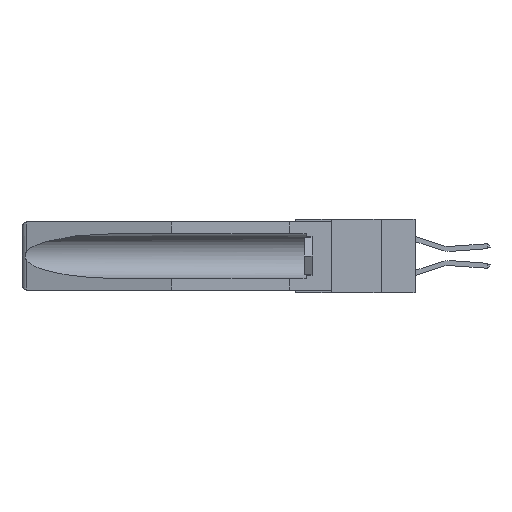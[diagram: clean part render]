
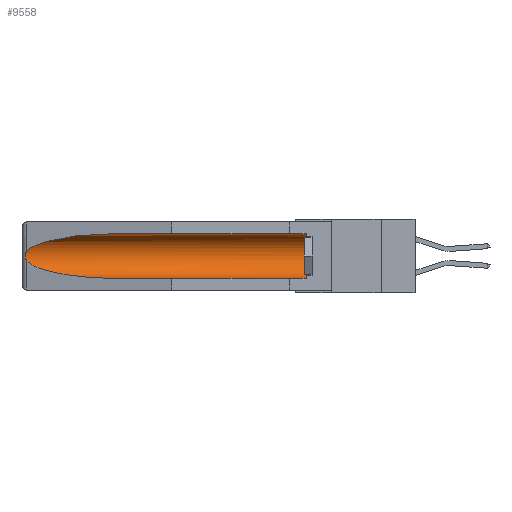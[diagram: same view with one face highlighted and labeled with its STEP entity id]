
A CAD part, left-side view. The second image highlights one B-rep face of the part: STEP entity #9558.
In plain terms, the highlighted cylindrical face has radius 2.857 mm (diameter 5.715 mm), a partial arc.
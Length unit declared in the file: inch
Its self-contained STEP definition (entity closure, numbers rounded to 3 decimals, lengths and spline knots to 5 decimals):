
#651 = ORIENTED_EDGE ( 'NONE', *, *, #10218, .F. ) ;
#733 = CIRCLE ( 'NONE', #18946, 0.1125 ) ;
#975 = CARTESIAN_POINT ( 'NONE',  ( 0.155, 1.07973, -0.059 ) ) ;
#1081 = CARTESIAN_POINT ( 'NONE',  ( 0.155, -0.30754, -0.1715 ) ) ;
#1108 = CARTESIAN_POINT ( 'NONE',  ( 0.155, 0.126, -0.284 ) ) ;
#1330 = VECTOR ( 'NONE', #5319, 39.37008 ) ;
#1684 = VERTEX_POINT ( 'NONE', #7099 ) ;
#2034 = CARTESIAN_POINT ( 'NONE',  ( 0.26537, 1.52718, -0.19328 ) ) ;
#2646 = DIRECTION ( 'NONE',  ( 0., 0., 1. ) ) ;
#2997 = CARTESIAN_POINT ( 'NONE',  ( 0.155, 0.126, -0.1715 ) ) ;
#3267 = EDGE_LOOP ( 'NONE', ( #19326, #18221, #10619, #651, #4637, #14459 ) ) ;
#3808 = CARTESIAN_POINT ( 'NONE',  ( 0.26537, 1.52718, -0.14972 ) ) ;
#3849 = DIRECTION ( 'NONE',  ( 0., 1., 0. ) ) ;
#4159 = EDGE_CURVE ( 'NONE', #10867, #6230, #10874, .T. ) ;
#4367 = CARTESIAN_POINT ( 'NONE',  ( 0.2675, 1.53308, -0.16763 ) ) ;
#4631 = DIRECTION ( 'NONE',  ( 0., 0., 1. ) ) ;
#4637 = ORIENTED_EDGE ( 'NONE', *, *, #15136, .T. ) ;
#5319 = DIRECTION ( 'NONE',  ( 0., 1., 0. ) ) ;
#5384 = CARTESIAN_POINT ( 'NONE',  ( 0.155, 1.07973, -0.059 ) ) ;
#5435 = EDGE_CURVE ( 'NONE', #6230, #8891, #6305, .T. ) ;
#5699 = CARTESIAN_POINT ( 'NONE',  ( 0.21114, 1.30732, -0.059 ) ) ;
#6230 = VERTEX_POINT ( 'NONE', #3808 ) ;
#6305 = B_SPLINE_CURVE_WITH_KNOTS ( 'NONE', 3,
 ( #15236, #7672, #13811, #8909, #4367, #15377, #16901, #19942, #10525, #20005 ),
 .UNSPECIFIED., .F., .F.,
 ( 4, 2, 2, 2, 4 ),
 ( 0., 0.00029, 0.00058, 0.00087, 0.00117 ),
 .UNSPECIFIED. ) ;
#7099 = CARTESIAN_POINT ( 'NONE',  ( 0.155, 0.126, -0.059 ) ) ;
#7160 = CARTESIAN_POINT ( 'NONE',  ( 0.155, -0.30754, -0.284 ) ) ;
#7672 = CARTESIAN_POINT ( 'NONE',  ( 0.26597, 1.52961, -0.15275 ) ) ;
#7878 = VERTEX_POINT ( 'NONE', #1108 ) ;
#8292 = CARTESIAN_POINT ( 'NONE',  ( 0.155, -0.30754, -0.059 ) ) ;
#8573 = CYLINDRICAL_SURFACE ( 'NONE', #11892, 0.1125 ) ;
#8720 =( BOUNDED_CURVE ( )  B_SPLINE_CURVE ( 3, ( #2034, #14272, #9805, #17841 ),
 .UNSPECIFIED., .F., .F. ) 
 B_SPLINE_CURVE_WITH_KNOTS ( ( 4, 4 ),
 ( 0.1948, 1.5708 ),
 .UNSPECIFIED. ) 
 CURVE ( )  GEOMETRIC_REPRESENTATION_ITEM ( )  RATIONAL_B_SPLINE_CURVE ( ( 1., 0.848, 0.848, 1. ) ) 
 REPRESENTATION_ITEM ( '' )  );
#8891 = VERTEX_POINT ( 'NONE', #19008 ) ;
#8909 = CARTESIAN_POINT ( 'NONE',  ( 0.2673, 1.5327, -0.16383 ) ) ;
#9558 = ADVANCED_FACE ( 'NONE', ( #14722 ), #8573, .F. ) ;
#9805 = CARTESIAN_POINT ( 'NONE',  ( 0.21114, 1.30732, -0.284 ) ) ;
#10205 = LINE ( 'NONE', #8292, #1330 ) ;
#10218 = EDGE_CURVE ( 'NONE', #7878, #10539, #19918, .T. ) ;
#10525 = CARTESIAN_POINT ( 'NONE',  ( 0.26597, 1.5296, -0.19026 ) ) ;
#10539 = VERTEX_POINT ( 'NONE', #16199 ) ;
#10619 = ORIENTED_EDGE ( 'NONE', *, *, #16459, .T. ) ;
#10867 = VERTEX_POINT ( 'NONE', #5384 ) ;
#10874 =( BOUNDED_CURVE ( )  B_SPLINE_CURVE ( 3, ( #975, #5699, #19913, #13640 ),
 .UNSPECIFIED., .F., .F. ) 
 B_SPLINE_CURVE_WITH_KNOTS ( ( 4, 4 ),
 ( 4.71239, 6.08839 ),
 .UNSPECIFIED. ) 
 CURVE ( )  GEOMETRIC_REPRESENTATION_ITEM ( )  RATIONAL_B_SPLINE_CURVE ( ( 1., 0.848, 0.848, 1. ) ) 
 REPRESENTATION_ITEM ( '' )  );
#11892 = AXIS2_PLACEMENT_3D ( 'NONE', #1081, #18478, #2646 ) ;
#11923 = VECTOR ( 'NONE', #3849, 39.37008 ) ;
#12382 = EDGE_CURVE ( 'NONE', #1684, #10867, #10205, .T. ) ;
#12521 = DIRECTION ( 'NONE',  ( 0., -1., 0. ) ) ;
#13640 = CARTESIAN_POINT ( 'NONE',  ( 0.26537, 1.52718, -0.14972 ) ) ;
#13811 = CARTESIAN_POINT ( 'NONE',  ( 0.26654, 1.53092, -0.15636 ) ) ;
#14272 = CARTESIAN_POINT ( 'NONE',  ( 0.25451, 1.48313, -0.24835 ) ) ;
#14459 = ORIENTED_EDGE ( 'NONE', *, *, #12382, .T. ) ;
#14722 = FACE_OUTER_BOUND ( 'NONE', #3267, .T. ) ;
#15136 = EDGE_CURVE ( 'NONE', #7878, #1684, #733, .T. ) ;
#15236 = CARTESIAN_POINT ( 'NONE',  ( 0.26537, 1.52718, -0.14972 ) ) ;
#15377 = CARTESIAN_POINT ( 'NONE',  ( 0.2675, 1.53308, -0.17534 ) ) ;
#16199 = CARTESIAN_POINT ( 'NONE',  ( 0.155, 1.07973, -0.284 ) ) ;
#16459 = EDGE_CURVE ( 'NONE', #8891, #10539, #8720, .T. ) ;
#16901 = CARTESIAN_POINT ( 'NONE',  ( 0.2673, 1.53269, -0.17917 ) ) ;
#17841 = CARTESIAN_POINT ( 'NONE',  ( 0.155, 1.07973, -0.284 ) ) ;
#18221 = ORIENTED_EDGE ( 'NONE', *, *, #5435, .T. ) ;
#18478 = DIRECTION ( 'NONE',  ( 0., 1., 0. ) ) ;
#18946 = AXIS2_PLACEMENT_3D ( 'NONE', #2997, #12521, #4631 ) ;
#19008 = CARTESIAN_POINT ( 'NONE',  ( 0.26537, 1.52718, -0.19328 ) ) ;
#19326 = ORIENTED_EDGE ( 'NONE', *, *, #4159, .T. ) ;
#19913 = CARTESIAN_POINT ( 'NONE',  ( 0.25451, 1.48313, -0.09465 ) ) ;
#19918 = LINE ( 'NONE', #7160, #11923 ) ;
#19942 = CARTESIAN_POINT ( 'NONE',  ( 0.26655, 1.53094, -0.18657 ) ) ;
#20005 = CARTESIAN_POINT ( 'NONE',  ( 0.26537, 1.52718, -0.19328 ) ) ;
